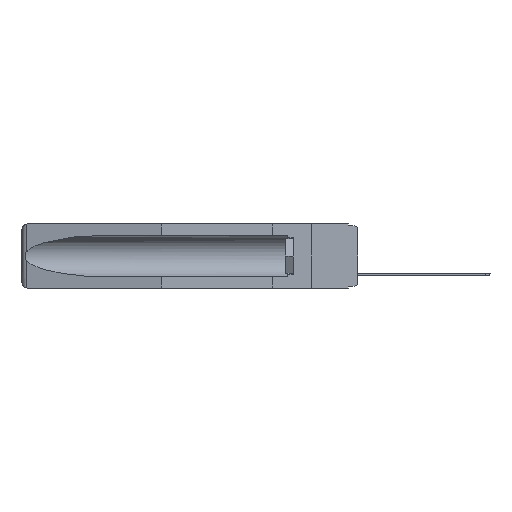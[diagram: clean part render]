
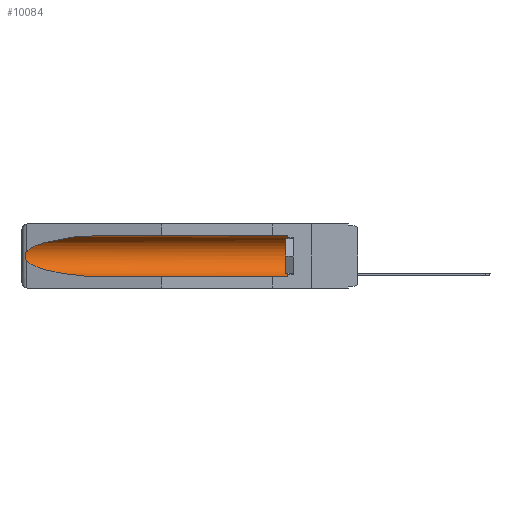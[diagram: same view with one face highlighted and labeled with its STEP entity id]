
A CAD part, left-side view. The second image highlights one B-rep face of the part: STEP entity #10084.
In plain terms, the highlighted cylindrical face has radius 2.857 mm (diameter 5.715 mm), a partial arc.
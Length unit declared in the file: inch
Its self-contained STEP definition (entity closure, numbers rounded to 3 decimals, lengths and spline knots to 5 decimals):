
#143 = CARTESIAN_POINT ( 'NONE',  ( 0.21114, 1.30732, -0.059 ) ) ;
#1520 = DIRECTION ( 'NONE',  ( 0., 1., 0. ) ) ;
#1591 = ORIENTED_EDGE ( 'NONE', *, *, #20687, .T. ) ;
#1884 = CYLINDRICAL_SURFACE ( 'NONE', #7818, 0.1125 ) ;
#2111 = FACE_OUTER_BOUND ( 'NONE', #2754, .T. ) ;
#2221 = EDGE_CURVE ( 'NONE', #12183, #3683, #13021, .T. ) ;
#2357 = CARTESIAN_POINT ( 'NONE',  ( 0.155, 1.07973, -0.059 ) ) ;
#2648 =( BOUNDED_CURVE ( )  B_SPLINE_CURVE ( 3, ( #18379, #18494, #11521, #16806 ),
 .UNSPECIFIED., .F., .T. ) 
 B_SPLINE_CURVE_WITH_KNOTS ( ( 4, 4 ),
 ( 0.1948, 1.5708 ),
 .UNSPECIFIED. ) 
 CURVE ( )  GEOMETRIC_REPRESENTATION_ITEM ( )  RATIONAL_B_SPLINE_CURVE ( ( 1., 0.848, 0.848, 1. ) ) 
 REPRESENTATION_ITEM ( '' )  );
#2754 = EDGE_LOOP ( 'NONE', ( #20916, #14087, #1591, #9156, #7769, #8497 ) ) ;
#3152 = AXIS2_PLACEMENT_3D ( 'NONE', #3398, #8479, #3167 ) ;
#3167 = DIRECTION ( 'NONE',  ( 0., 0., 1. ) ) ;
#3215 = CARTESIAN_POINT ( 'NONE',  ( 0.26537, 1.52718, -0.19328 ) ) ;
#3331 = CARTESIAN_POINT ( 'NONE',  ( 0.26655, 1.53094, -0.18657 ) ) ;
#3398 = CARTESIAN_POINT ( 'NONE',  ( 0.155, 0.126, -0.1715 ) ) ;
#3683 = VERTEX_POINT ( 'NONE', #13802 ) ;
#5141 = CARTESIAN_POINT ( 'NONE',  ( 0.26654, 1.53092, -0.15636 ) ) ;
#5154 = VERTEX_POINT ( 'NONE', #18144 ) ;
#6167 = CARTESIAN_POINT ( 'NONE',  ( 0.26537, 1.52718, -0.14972 ) ) ;
#6506 = CARTESIAN_POINT ( 'NONE',  ( 0.2675, 1.53308, -0.16763 ) ) ;
#6618 = CARTESIAN_POINT ( 'NONE',  ( 0.2673, 1.5327, -0.16383 ) ) ;
#7769 = ORIENTED_EDGE ( 'NONE', *, *, #11271, .T. ) ;
#7818 = AXIS2_PLACEMENT_3D ( 'NONE', #19259, #9008, #13611 ) ;
#7851 = CIRCLE ( 'NONE', #3152, 0.1125 ) ;
#8193 = CARTESIAN_POINT ( 'NONE',  ( 0.26597, 1.5296, -0.19026 ) ) ;
#8479 = DIRECTION ( 'NONE',  ( 0., -1., 0. ) ) ;
#8497 = ORIENTED_EDGE ( 'NONE', *, *, #15580, .T. ) ;
#8629 = CARTESIAN_POINT ( 'NONE',  ( 0.2675, 1.53308, -0.17534 ) ) ;
#9008 = DIRECTION ( 'NONE',  ( 0., 1., 0. ) ) ;
#9156 = ORIENTED_EDGE ( 'NONE', *, *, #2221, .F. ) ;
#9799 = CARTESIAN_POINT ( 'NONE',  ( 0.26537, 1.52718, -0.19328 ) ) ;
#10084 = ADVANCED_FACE ( 'NONE', ( #2111 ), #1884, .F. ) ;
#10521 = CARTESIAN_POINT ( 'NONE',  ( 0.26537, 1.52718, -0.14972 ) ) ;
#10653 = CARTESIAN_POINT ( 'NONE',  ( 0.155, 0.126, -0.284 ) ) ;
#10844 = VECTOR ( 'NONE', #16197, 39.37008 ) ;
#11271 = EDGE_CURVE ( 'NONE', #12183, #21213, #7851, .T. ) ;
#11423 = VERTEX_POINT ( 'NONE', #2357 ) ;
#11521 = CARTESIAN_POINT ( 'NONE',  ( 0.21114, 1.30732, -0.284 ) ) ;
#12012 = CARTESIAN_POINT ( 'NONE',  ( 0.2673, 1.53269, -0.17917 ) ) ;
#12183 = VERTEX_POINT ( 'NONE', #10653 ) ;
#12237 = B_SPLINE_CURVE_WITH_KNOTS ( 'NONE', 3,
 ( #6167, #15164, #5141, #6618, #6506, #8629, #12012, #3331, #8193, #3215 ),
 .UNSPECIFIED., .F., .F.,
 ( 4, 2, 2, 2, 4 ),
 ( 0., 0.00029, 0.00058, 0.00087, 0.00117 ),
 .UNSPECIFIED. ) ;
#12603 = VECTOR ( 'NONE', #1520, 39.37008 ) ;
#13021 = LINE ( 'NONE', #21720, #12603 ) ;
#13611 = DIRECTION ( 'NONE',  ( 0., 0., 1. ) ) ;
#13802 = CARTESIAN_POINT ( 'NONE',  ( 0.155, 1.07973, -0.284 ) ) ;
#14087 = ORIENTED_EDGE ( 'NONE', *, *, #19826, .T. ) ;
#14885 =( BOUNDED_CURVE ( )  B_SPLINE_CURVE ( 3, ( #17490, #143, #20984, #10521 ),
 .UNSPECIFIED., .F., .T. ) 
 B_SPLINE_CURVE_WITH_KNOTS ( ( 4, 4 ),
 ( 4.71239, 6.08839 ),
 .UNSPECIFIED. ) 
 CURVE ( )  GEOMETRIC_REPRESENTATION_ITEM ( )  RATIONAL_B_SPLINE_CURVE ( ( 1., 0.848, 0.848, 1. ) ) 
 REPRESENTATION_ITEM ( '' )  );
#15164 = CARTESIAN_POINT ( 'NONE',  ( 0.26597, 1.52961, -0.15275 ) ) ;
#15580 = EDGE_CURVE ( 'NONE', #21213, #11423, #21278, .T. ) ;
#16197 = DIRECTION ( 'NONE',  ( 0., 1., 0. ) ) ;
#16806 = CARTESIAN_POINT ( 'NONE',  ( 0.155, 1.07973, -0.284 ) ) ;
#17490 = CARTESIAN_POINT ( 'NONE',  ( 0.155, 1.07973, -0.059 ) ) ;
#17994 = VERTEX_POINT ( 'NONE', #9799 ) ;
#18144 = CARTESIAN_POINT ( 'NONE',  ( 0.26537, 1.52718, -0.14972 ) ) ;
#18379 = CARTESIAN_POINT ( 'NONE',  ( 0.26537, 1.52718, -0.19328 ) ) ;
#18494 = CARTESIAN_POINT ( 'NONE',  ( 0.25451, 1.48313, -0.24835 ) ) ;
#18823 = CARTESIAN_POINT ( 'NONE',  ( 0.155, 0.126, -0.059 ) ) ;
#19159 = EDGE_CURVE ( 'NONE', #11423, #5154, #14885, .T. ) ;
#19259 = CARTESIAN_POINT ( 'NONE',  ( 0.155, -0.30754, -0.1715 ) ) ;
#19826 = EDGE_CURVE ( 'NONE', #5154, #17994, #12237, .T. ) ;
#20687 = EDGE_CURVE ( 'NONE', #17994, #3683, #2648, .T. ) ;
#20916 = ORIENTED_EDGE ( 'NONE', *, *, #19159, .T. ) ;
#20984 = CARTESIAN_POINT ( 'NONE',  ( 0.25451, 1.48313, -0.09465 ) ) ;
#21213 = VERTEX_POINT ( 'NONE', #18823 ) ;
#21278 = LINE ( 'NONE', #21615, #10844 ) ;
#21615 = CARTESIAN_POINT ( 'NONE',  ( 0.155, -0.30754, -0.059 ) ) ;
#21720 = CARTESIAN_POINT ( 'NONE',  ( 0.155, -0.30754, -0.284 ) ) ;
